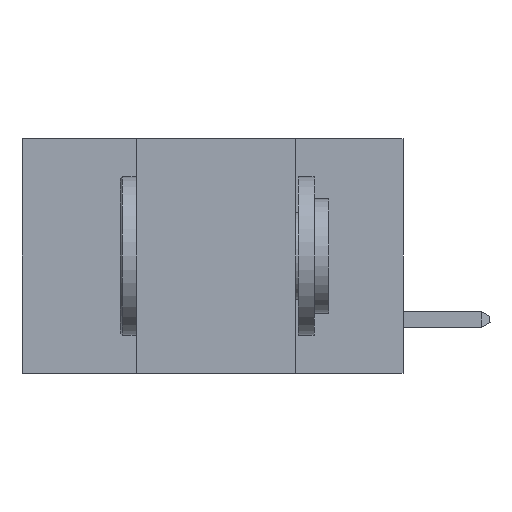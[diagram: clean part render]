
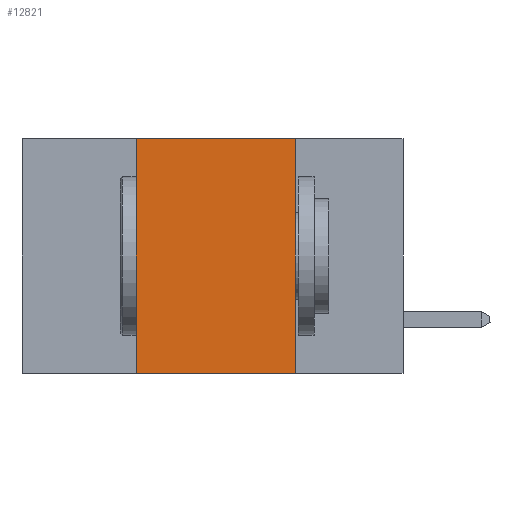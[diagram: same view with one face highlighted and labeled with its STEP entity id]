
A CAD part, left-side view. The second image highlights one B-rep face of the part: STEP entity #12821.
In plain terms, the highlighted planar face has unit normal (-1, 0, 0).
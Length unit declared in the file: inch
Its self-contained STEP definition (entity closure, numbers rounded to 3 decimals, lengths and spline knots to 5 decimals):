
#301 = DIRECTION ( 'NONE',  ( 0., -1., 0. ) ) ;
#481 = FACE_OUTER_BOUND ( 'NONE', #22278, .T. ) ;
#1230 = ORIENTED_EDGE ( 'NONE', *, *, #5308, .T. ) ;
#2999 = VECTOR ( 'NONE', #38005, 39.37008 ) ;
#3089 = VERTEX_POINT ( 'NONE', #19339 ) ;
#3396 = LINE ( 'NONE', #7425, #8324 ) ;
#5308 = EDGE_CURVE ( 'NONE', #41165, #24351, #6833, .T. ) ;
#5372 = CARTESIAN_POINT ( 'NONE',  ( 0., 0.42, 0. ) ) ;
#5407 = DIRECTION ( 'NONE',  ( 0., -1., 0. ) ) ;
#6833 = LINE ( 'NONE', #23582, #45138 ) ;
#7425 = CARTESIAN_POINT ( 'NONE',  ( 0., 0.17, 0. ) ) ;
#8324 = VECTOR ( 'NONE', #15656, 39.37008 ) ;
#8658 = CARTESIAN_POINT ( 'NONE',  ( 0., 0.6, 0. ) ) ;
#10831 = DIRECTION ( 'NONE',  ( 0., 0., -1. ) ) ;
#12821 = ADVANCED_FACE ( 'NONE', ( #481 ), #41604, .F. ) ;
#13197 = EDGE_CURVE ( 'NONE', #3089, #36547, #15894, .T. ) ;
#15656 = DIRECTION ( 'NONE',  ( 0., 0., -1. ) ) ;
#15894 = LINE ( 'NONE', #8658, #21892 ) ;
#18530 = CARTESIAN_POINT ( 'NONE',  ( 0., 0.17, 0. ) ) ;
#19339 = CARTESIAN_POINT ( 'NONE',  ( 0., 0.42, 0. ) ) ;
#21078 = EDGE_CURVE ( 'NONE', #36547, #24351, #3396, .T. ) ;
#21768 = ORIENTED_EDGE ( 'NONE', *, *, #21078, .F. ) ;
#21892 = VECTOR ( 'NONE', #5407, 39.37008 ) ;
#22278 = EDGE_LOOP ( 'NONE', ( #21768, #25692, #34903, #1230 ) ) ;
#23582 = CARTESIAN_POINT ( 'NONE',  ( 0., 0.6, -0.37 ) ) ;
#24351 = VERTEX_POINT ( 'NONE', #42985 ) ;
#25692 = ORIENTED_EDGE ( 'NONE', *, *, #13197, .F. ) ;
#28876 = AXIS2_PLACEMENT_3D ( 'NONE', #29740, #40396, #10831 ) ;
#29740 = CARTESIAN_POINT ( 'NONE',  ( 0., 0.6, 0. ) ) ;
#32455 = CARTESIAN_POINT ( 'NONE',  ( 0., 0.42, -0.37 ) ) ;
#33723 = LINE ( 'NONE', #5372, #2999 ) ;
#34903 = ORIENTED_EDGE ( 'NONE', *, *, #35607, .F. ) ;
#35607 = EDGE_CURVE ( 'NONE', #41165, #3089, #33723, .T. ) ;
#36547 = VERTEX_POINT ( 'NONE', #18530 ) ;
#38005 = DIRECTION ( 'NONE',  ( 0., 0., 1. ) ) ;
#40396 = DIRECTION ( 'NONE',  ( 1., 0., 0. ) ) ;
#41165 = VERTEX_POINT ( 'NONE', #32455 ) ;
#41604 = PLANE ( 'NONE',  #28876 ) ;
#42985 = CARTESIAN_POINT ( 'NONE',  ( 0., 0.17, -0.37 ) ) ;
#45138 = VECTOR ( 'NONE', #301, 39.37008 ) ;
